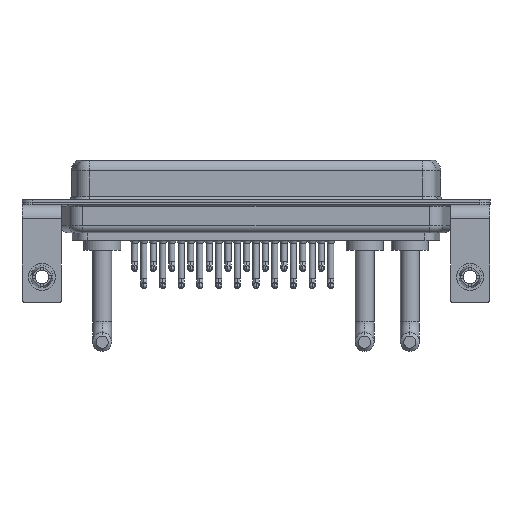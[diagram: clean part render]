
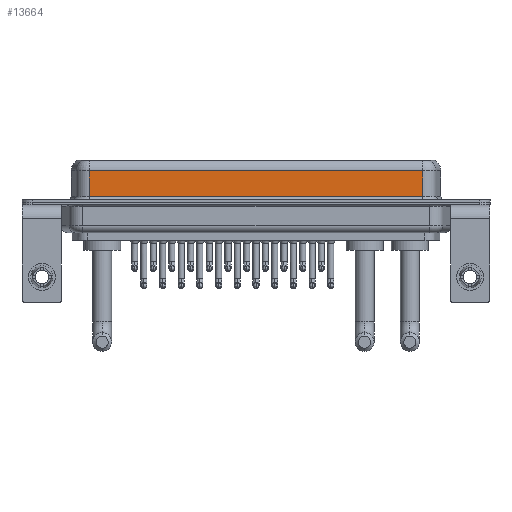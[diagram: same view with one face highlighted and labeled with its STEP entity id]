
A CAD part, front view. The second image highlights one B-rep face of the part: STEP entity #13664.
In plain terms, the highlighted planar face has unit normal (0, -1, 0).
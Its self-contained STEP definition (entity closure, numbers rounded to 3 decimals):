
#1402 = CARTESIAN_POINT ( 'NONE',  ( 7.038, -3.95, 6.4 ) ) ;
#1530 = CARTESIAN_POINT ( 'NONE',  ( 56.462, -3.95, 6.4 ) ) ;
#1641 = CARTESIAN_POINT ( 'NONE',  ( 7.038, -3.95, 4.65 ) ) ;
#2595 = EDGE_CURVE ( 'NONE', #22121, #5380, #5395, .T. ) ;
#3423 = ORIENTED_EDGE ( 'NONE', *, *, #2595, .F. ) ;
#5380 = VERTEX_POINT ( 'NONE', #12667 ) ;
#5395 = LINE ( 'NONE', #1530, #14799 ) ;
#5653 = LINE ( 'NONE', #1402, #21663 ) ;
#6475 = LINE ( 'NONE', #14555, #14530 ) ;
#7400 = DIRECTION ( 'NONE',  ( 0., 0., -1. ) ) ;
#8338 = VERTEX_POINT ( 'NONE', #1641 ) ;
#8952 = ORIENTED_EDGE ( 'NONE', *, *, #21101, .T. ) ;
#9392 = DIRECTION ( 'NONE',  ( 0., 1., 0. ) ) ;
#9657 = DIRECTION ( 'NONE',  ( 0., 0., -1. ) ) ;
#10145 = LINE ( 'NONE', #22448, #25760 ) ;
#11638 = FACE_OUTER_BOUND ( 'NONE', #23914, .T. ) ;
#11887 = DIRECTION ( 'NONE',  ( 1., 0., 0. ) ) ;
#12667 = CARTESIAN_POINT ( 'NONE',  ( 56.462, -3.95, 0.9 ) ) ;
#13222 = DIRECTION ( 'NONE',  ( 0., 0., 1. ) ) ;
#13664 = ADVANCED_FACE ( 'NONE', ( #11638 ), #19712, .F. ) ;
#14530 = VECTOR ( 'NONE', #18672, 1000. ) ;
#14555 = CARTESIAN_POINT ( 'NONE',  ( 56.462, -3.95, 4.65 ) ) ;
#14799 = VECTOR ( 'NONE', #9657, 1000. ) ;
#14931 = EDGE_CURVE ( 'NONE', #8338, #24477, #5653, .T. ) ;
#16088 = EDGE_CURVE ( 'NONE', #22121, #8338, #6475, .T. ) ;
#18672 = DIRECTION ( 'NONE',  ( -1., 0., 0. ) ) ;
#18720 = CARTESIAN_POINT ( 'NONE',  ( 7.038, -3.95, 0.9 ) ) ;
#19276 = AXIS2_PLACEMENT_3D ( 'NONE', #19448, #9392, #13222 ) ;
#19448 = CARTESIAN_POINT ( 'NONE',  ( 56.462, -3.95, 6.4 ) ) ;
#19712 = PLANE ( 'NONE',  #19276 ) ;
#21101 = EDGE_CURVE ( 'NONE', #24477, #5380, #10145, .T. ) ;
#21663 = VECTOR ( 'NONE', #7400, 1000. ) ;
#21877 = ORIENTED_EDGE ( 'NONE', *, *, #16088, .T. ) ;
#22121 = VERTEX_POINT ( 'NONE', #24469 ) ;
#22448 = CARTESIAN_POINT ( 'NONE',  ( 56.462, -3.95, 0.9 ) ) ;
#23794 = ORIENTED_EDGE ( 'NONE', *, *, #14931, .T. ) ;
#23914 = EDGE_LOOP ( 'NONE', ( #3423, #21877, #23794, #8952 ) ) ;
#24469 = CARTESIAN_POINT ( 'NONE',  ( 56.462, -3.95, 4.65 ) ) ;
#24477 = VERTEX_POINT ( 'NONE', #18720 ) ;
#25760 = VECTOR ( 'NONE', #11887, 1000. ) ;
